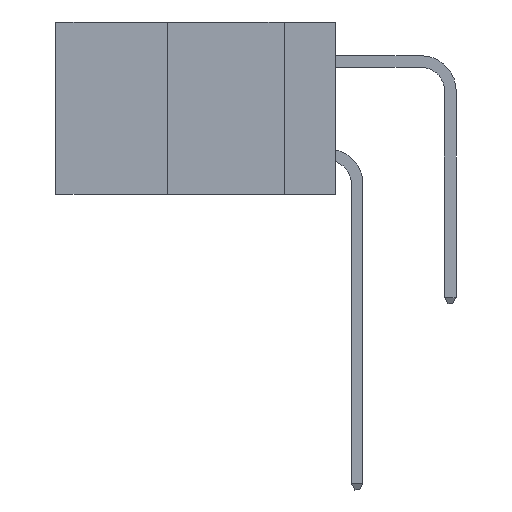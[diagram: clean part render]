
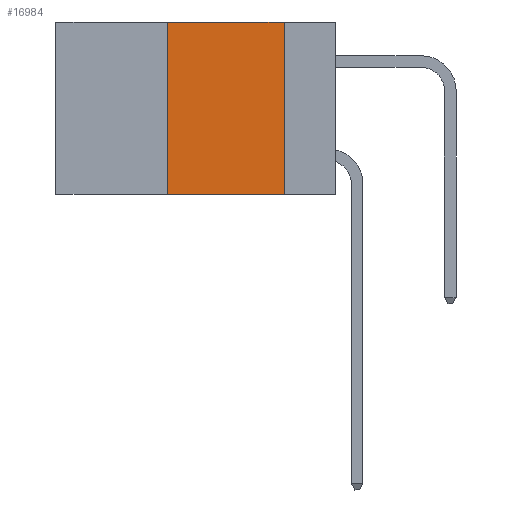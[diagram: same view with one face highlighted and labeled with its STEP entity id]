
A CAD part, left-side view. The second image highlights one B-rep face of the part: STEP entity #16984.
In plain terms, the highlighted planar face has unit normal (-1, 0, 0).
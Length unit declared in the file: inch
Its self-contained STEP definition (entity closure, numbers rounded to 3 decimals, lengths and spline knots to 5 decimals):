
#224 = VERTEX_POINT ( 'NONE', #19275 ) ;
#442 = EDGE_CURVE ( 'NONE', #17648, #8127, #19537, .T. ) ;
#914 = DIRECTION ( 'NONE',  ( 1., 0., 0. ) ) ;
#2757 = VECTOR ( 'NONE', #9854, 39.37008 ) ;
#2821 = LINE ( 'NONE', #16882, #14550 ) ;
#2829 = CARTESIAN_POINT ( 'NONE',  ( 0., 0.11, -0.37 ) ) ;
#5350 = VECTOR ( 'NONE', #24106, 39.37008 ) ;
#8127 = VERTEX_POINT ( 'NONE', #10118 ) ;
#8528 = LINE ( 'NONE', #22366, #5350 ) ;
#8935 = AXIS2_PLACEMENT_3D ( 'NONE', #23551, #914, #15208 ) ;
#9649 = DIRECTION ( 'NONE',  ( 0., 0., -1. ) ) ;
#9854 = DIRECTION ( 'NONE',  ( 0., -1., 0. ) ) ;
#10118 = CARTESIAN_POINT ( 'NONE',  ( 0., 0.11, 0. ) ) ;
#12424 = VERTEX_POINT ( 'NONE', #2829 ) ;
#13945 = ORIENTED_EDGE ( 'NONE', *, *, #24592, .F. ) ;
#14550 = VECTOR ( 'NONE', #24745, 39.37008 ) ;
#15208 = DIRECTION ( 'NONE',  ( 0., 0., -1. ) ) ;
#16828 = EDGE_CURVE ( 'NONE', #8127, #12424, #18908, .T. ) ;
#16882 = CARTESIAN_POINT ( 'NONE',  ( 0., 0.36, 0. ) ) ;
#16939 = ORIENTED_EDGE ( 'NONE', *, *, #442, .F. ) ;
#16984 = ADVANCED_FACE ( 'NONE', ( #17687 ), #21386, .F. ) ;
#17091 = EDGE_CURVE ( 'NONE', #224, #12424, #8528, .T. ) ;
#17352 = VECTOR ( 'NONE', #9649, 39.37008 ) ;
#17648 = VERTEX_POINT ( 'NONE', #21197 ) ;
#17687 = FACE_OUTER_BOUND ( 'NONE', #26278, .T. ) ;
#18267 = CARTESIAN_POINT ( 'NONE',  ( 0., 0.6, 0. ) ) ;
#18908 = LINE ( 'NONE', #24648, #17352 ) ;
#19275 = CARTESIAN_POINT ( 'NONE',  ( 0., 0.36, -0.37 ) ) ;
#19537 = LINE ( 'NONE', #18267, #2757 ) ;
#21197 = CARTESIAN_POINT ( 'NONE',  ( 0., 0.36, 0. ) ) ;
#21386 = PLANE ( 'NONE',  #8935 ) ;
#22090 = ORIENTED_EDGE ( 'NONE', *, *, #17091, .T. ) ;
#22366 = CARTESIAN_POINT ( 'NONE',  ( 0., 0.6, -0.37 ) ) ;
#23551 = CARTESIAN_POINT ( 'NONE',  ( 0., 0.6, 0. ) ) ;
#24106 = DIRECTION ( 'NONE',  ( 0., -1., 0. ) ) ;
#24312 = ORIENTED_EDGE ( 'NONE', *, *, #16828, .F. ) ;
#24592 = EDGE_CURVE ( 'NONE', #224, #17648, #2821, .T. ) ;
#24648 = CARTESIAN_POINT ( 'NONE',  ( 0., 0.11, 0. ) ) ;
#24745 = DIRECTION ( 'NONE',  ( 0., 0., 1. ) ) ;
#26278 = EDGE_LOOP ( 'NONE', ( #24312, #16939, #13945, #22090 ) ) ;
